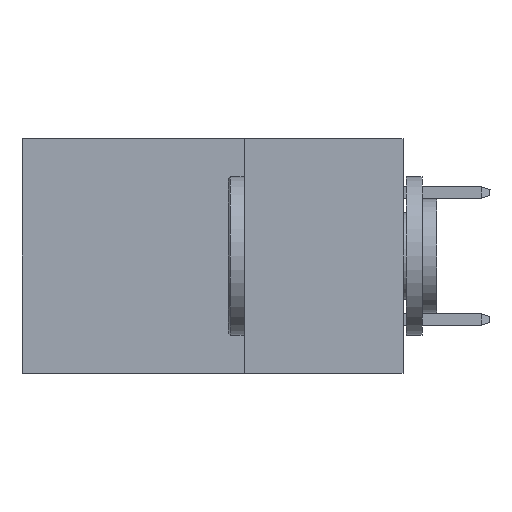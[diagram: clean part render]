
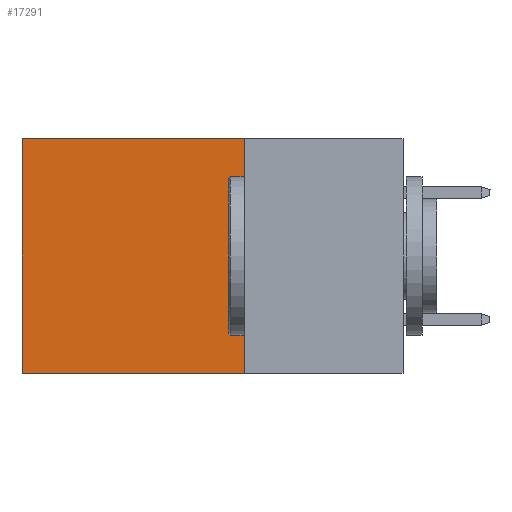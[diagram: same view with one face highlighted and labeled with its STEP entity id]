
A CAD part, left-side view. The second image highlights one B-rep face of the part: STEP entity #17291.
In plain terms, the highlighted planar face has unit normal (-1, 0, 0).
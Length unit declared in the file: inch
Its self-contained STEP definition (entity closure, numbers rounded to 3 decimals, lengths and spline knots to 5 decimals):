
#416 = LINE ( 'NONE', #20704, #4917 ) ;
#689 = CARTESIAN_POINT ( 'NONE',  ( 0.2875, 0.25, -0.37 ) ) ;
#1441 = EDGE_CURVE ( 'NONE', #17227, #3198, #416, .T. ) ;
#1476 = LINE ( 'NONE', #8376, #6330 ) ;
#2124 = EDGE_CURVE ( 'NONE', #8831, #2481, #1476, .T. ) ;
#2481 = VERTEX_POINT ( 'NONE', #689 ) ;
#3198 = VERTEX_POINT ( 'NONE', #17115 ) ;
#4121 = EDGE_LOOP ( 'NONE', ( #9672, #16971, #6583, #5053 ) ) ;
#4849 = PLANE ( 'NONE',  #5291 ) ;
#4917 = VECTOR ( 'NONE', #17677, 39.37008 ) ;
#5053 = ORIENTED_EDGE ( 'NONE', *, *, #12108, .T. ) ;
#5153 = CARTESIAN_POINT ( 'NONE',  ( 0.2875, 0.25, 0. ) ) ;
#5291 = AXIS2_PLACEMENT_3D ( 'NONE', #15325, #21715, #9875 ) ;
#6330 = VECTOR ( 'NONE', #18436, 39.37008 ) ;
#6583 = ORIENTED_EDGE ( 'NONE', *, *, #2124, .F. ) ;
#6816 = DIRECTION ( 'NONE',  ( 0., 1., 0. ) ) ;
#8376 = CARTESIAN_POINT ( 'NONE',  ( 0.2875, 0.25, 0. ) ) ;
#8831 = VERTEX_POINT ( 'NONE', #9858 ) ;
#9148 = EDGE_CURVE ( 'NONE', #2481, #3198, #20308, .T. ) ;
#9657 = CARTESIAN_POINT ( 'NONE',  ( 0.2875, 0.6, 0. ) ) ;
#9672 = ORIENTED_EDGE ( 'NONE', *, *, #1441, .T. ) ;
#9858 = CARTESIAN_POINT ( 'NONE',  ( 0.2875, 0.25, 0. ) ) ;
#9875 = DIRECTION ( 'NONE',  ( 0., 0., -1. ) ) ;
#12108 = EDGE_CURVE ( 'NONE', #8831, #17227, #18545, .T. ) ;
#13162 = CARTESIAN_POINT ( 'NONE',  ( 0.2875, 0.25, -0.37 ) ) ;
#15325 = CARTESIAN_POINT ( 'NONE',  ( 0.2875, 0.25, 0. ) ) ;
#16552 = FACE_OUTER_BOUND ( 'NONE', #4121, .T. ) ;
#16677 = VECTOR ( 'NONE', #20092, 39.37008 ) ;
#16971 = ORIENTED_EDGE ( 'NONE', *, *, #9148, .F. ) ;
#17115 = CARTESIAN_POINT ( 'NONE',  ( 0.2875, 0.6, -0.37 ) ) ;
#17227 = VERTEX_POINT ( 'NONE', #9657 ) ;
#17291 = ADVANCED_FACE ( 'NONE', ( #16552 ), #4849, .F. ) ;
#17677 = DIRECTION ( 'NONE',  ( 0., 0., -1. ) ) ;
#18436 = DIRECTION ( 'NONE',  ( 0., 0., -1. ) ) ;
#18545 = LINE ( 'NONE', #5153, #21097 ) ;
#20092 = DIRECTION ( 'NONE',  ( 0., 1., 0. ) ) ;
#20308 = LINE ( 'NONE', #13162, #16677 ) ;
#20704 = CARTESIAN_POINT ( 'NONE',  ( 0.2875, 0.6, 0. ) ) ;
#21097 = VECTOR ( 'NONE', #6816, 39.37008 ) ;
#21715 = DIRECTION ( 'NONE',  ( 1., 0., 0. ) ) ;
